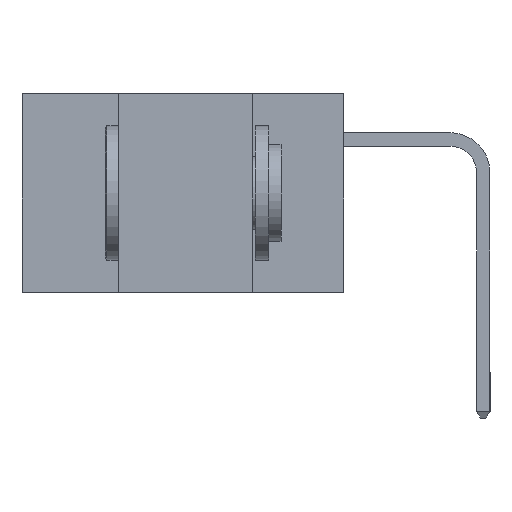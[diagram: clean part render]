
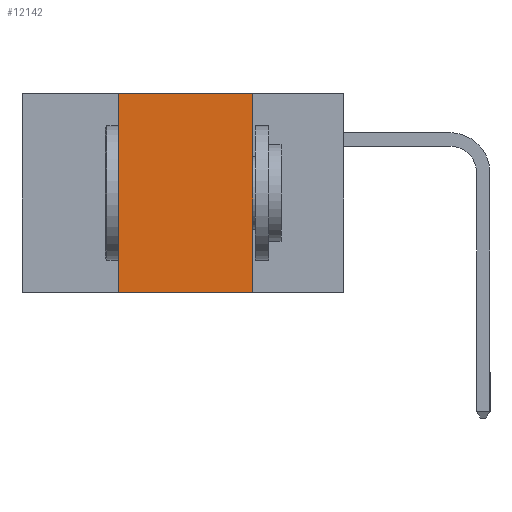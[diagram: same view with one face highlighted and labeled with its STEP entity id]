
A CAD part, left-side view. The second image highlights one B-rep face of the part: STEP entity #12142.
In plain terms, the highlighted planar face has unit normal (-1, 0, 0).
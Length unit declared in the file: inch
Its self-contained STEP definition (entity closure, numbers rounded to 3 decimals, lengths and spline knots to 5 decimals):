
#2396 = LINE ( 'NONE', #24754, #26361 ) ;
#2752 = CARTESIAN_POINT ( 'NONE',  ( 0., 0.17, -0.37 ) ) ;
#3639 = VERTEX_POINT ( 'NONE', #20235 ) ;
#4946 = EDGE_CURVE ( 'NONE', #17569, #11108, #7783, .T. ) ;
#5389 = EDGE_CURVE ( 'NONE', #3639, #10789, #16985, .T. ) ;
#5740 = DIRECTION ( 'NONE',  ( 0., 0., -1. ) ) ;
#7335 = DIRECTION ( 'NONE',  ( 0., 0., -1. ) ) ;
#7628 = CARTESIAN_POINT ( 'NONE',  ( 0., 0.6, 0. ) ) ;
#7783 = LINE ( 'NONE', #16106, #11702 ) ;
#9969 = EDGE_CURVE ( 'NONE', #10789, #17569, #2396, .T. ) ;
#10082 = CARTESIAN_POINT ( 'NONE',  ( 0., 0.17, 0. ) ) ;
#10789 = VERTEX_POINT ( 'NONE', #22638 ) ;
#11108 = VERTEX_POINT ( 'NONE', #2752 ) ;
#11187 = VECTOR ( 'NONE', #13964, 39.37008 ) ;
#11702 = VECTOR ( 'NONE', #5740, 39.37008 ) ;
#12142 = ADVANCED_FACE ( 'NONE', ( #18005 ), #26391, .F. ) ;
#13964 = DIRECTION ( 'NONE',  ( 0., -1., 0. ) ) ;
#14686 = CARTESIAN_POINT ( 'NONE',  ( 0., 0.42, -0.37 ) ) ;
#16106 = CARTESIAN_POINT ( 'NONE',  ( 0., 0.17, -0.37 ) ) ;
#16511 = VECTOR ( 'NONE', #25366, 39.37008 ) ;
#16590 = EDGE_CURVE ( 'NONE', #3639, #11108, #24084, .T. ) ;
#16985 = LINE ( 'NONE', #14686, #16511 ) ;
#17569 = VERTEX_POINT ( 'NONE', #10082 ) ;
#18005 = FACE_OUTER_BOUND ( 'NONE', #23910, .T. ) ;
#18019 = AXIS2_PLACEMENT_3D ( 'NONE', #7628, #21994, #7335 ) ;
#19206 = ORIENTED_EDGE ( 'NONE', *, *, #9969, .F. ) ;
#19733 = ORIENTED_EDGE ( 'NONE', *, *, #16590, .T. ) ;
#20235 = CARTESIAN_POINT ( 'NONE',  ( 0., 0.42, -0.37 ) ) ;
#21699 = DIRECTION ( 'NONE',  ( 0., -1., 0. ) ) ;
#21994 = DIRECTION ( 'NONE',  ( 1., 0., 0. ) ) ;
#22638 = CARTESIAN_POINT ( 'NONE',  ( 0., 0.42, 0. ) ) ;
#22901 = ORIENTED_EDGE ( 'NONE', *, *, #5389, .F. ) ;
#23593 = ORIENTED_EDGE ( 'NONE', *, *, #4946, .F. ) ;
#23910 = EDGE_LOOP ( 'NONE', ( #23593, #19206, #22901, #19733 ) ) ;
#24084 = LINE ( 'NONE', #24368, #11187 ) ;
#24368 = CARTESIAN_POINT ( 'NONE',  ( 0., 0.6, -0.37 ) ) ;
#24754 = CARTESIAN_POINT ( 'NONE',  ( 0., 0.6, 0. ) ) ;
#25366 = DIRECTION ( 'NONE',  ( 0., 0., 1. ) ) ;
#26361 = VECTOR ( 'NONE', #21699, 39.37008 ) ;
#26391 = PLANE ( 'NONE',  #18019 ) ;
